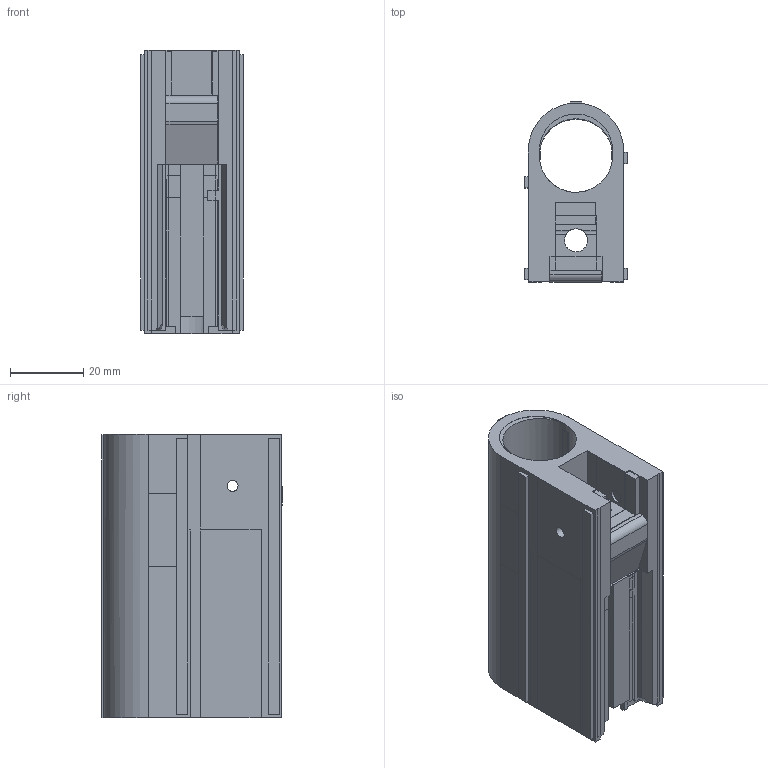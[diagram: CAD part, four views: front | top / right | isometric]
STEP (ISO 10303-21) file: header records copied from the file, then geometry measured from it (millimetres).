
FILE_DESCRIPTION(('FreeCAD Model'),'2;1');
FILE_NAME('ap9 bolt housing 2020.step','2020-04-04T17:34:47',('Author'),(''), 'Open CASCADE STEP processor 6.8','FreeCAD','Unknown');
FILE_SCHEMA(('AUTOMOTIVE_DESIGN_CC2 { 1 2 10303 214 -1 1 5 4 }'));
Length unit declared in the file: millimetre
Products named in the file (1): Pad008
Bounding box: 28 x 49.1 x 77.19 mm (x, y, z)
Volume: 43766.7 mm3; surface area: 21621 mm2
Topology: 1 solids, 3 shells, 252 faces, 692 edges, 449 vertices
Faces by surface type: plane 233, cylinder 19
Full cylindrical faces by diameter (mm): 2.968 x2, 3 x1, 3.566 x1, 6.34 x1, 20 x1
Entity records: 17929 total; most frequent: CARTESIAN_POINT 4454, DIRECTION 2372, LINE 1627, VECTOR 1627, ORIENTED_EDGE 1384, PCURVE 1384, DEFINITIONAL_REPRESENTATION 1384, EDGE_CURVE 692
